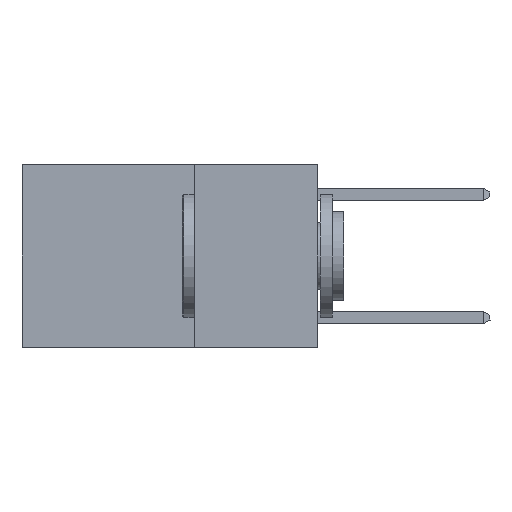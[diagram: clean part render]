
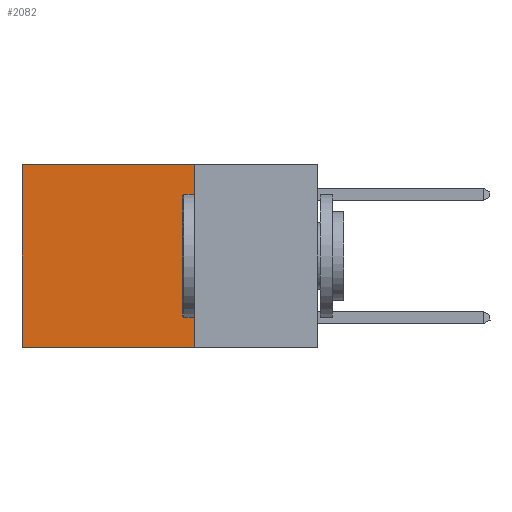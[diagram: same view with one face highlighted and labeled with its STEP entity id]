
A CAD part, left-side view. The second image highlights one B-rep face of the part: STEP entity #2082.
In plain terms, the highlighted planar face has unit normal (-1, 0, 0).
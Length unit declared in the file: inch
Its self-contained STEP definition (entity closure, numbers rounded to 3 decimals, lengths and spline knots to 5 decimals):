
#251 = DIRECTION ( 'NONE',  ( 0., 0., -1. ) ) ;
#356 = CARTESIAN_POINT ( 'NONE',  ( 0.2625, 0.6, 0. ) ) ;
#1364 = ORIENTED_EDGE ( 'NONE', *, *, #13671, .T. ) ;
#1718 = AXIS2_PLACEMENT_3D ( 'NONE', #10897, #9936, #9762 ) ;
#1828 = ORIENTED_EDGE ( 'NONE', *, *, #12898, .F. ) ;
#2082 = ADVANCED_FACE ( 'NONE', ( #7161 ), #16792, .F. ) ;
#2139 = EDGE_CURVE ( 'NONE', #4637, #15109, #13131, .T. ) ;
#2626 = EDGE_CURVE ( 'NONE', #5519, #4915, #13304, .T. ) ;
#2688 = VECTOR ( 'NONE', #3505, 39.37008 ) ;
#2850 = CARTESIAN_POINT ( 'NONE',  ( 0.2625, 0.25, 0. ) ) ;
#3505 = DIRECTION ( 'NONE',  ( 0., 1., 0. ) ) ;
#3754 = DIRECTION ( 'NONE',  ( 0., 1., 0. ) ) ;
#3879 = CARTESIAN_POINT ( 'NONE',  ( 0.2625, 0.25, 0. ) ) ;
#4637 = VERTEX_POINT ( 'NONE', #8286 ) ;
#4915 = VERTEX_POINT ( 'NONE', #356 ) ;
#5519 = VERTEX_POINT ( 'NONE', #2850 ) ;
#5584 = VECTOR ( 'NONE', #251, 39.37008 ) ;
#7161 = FACE_OUTER_BOUND ( 'NONE', #12252, .T. ) ;
#8125 = CARTESIAN_POINT ( 'NONE',  ( 0.2625, 0.6, -0.37 ) ) ;
#8286 = CARTESIAN_POINT ( 'NONE',  ( 0.2625, 0.25, -0.37 ) ) ;
#8288 = VECTOR ( 'NONE', #12950, 39.37008 ) ;
#9135 = LINE ( 'NONE', #14086, #5584 ) ;
#9658 = VECTOR ( 'NONE', #3754, 39.37008 ) ;
#9762 = DIRECTION ( 'NONE',  ( 0., 0., -1. ) ) ;
#9936 = DIRECTION ( 'NONE',  ( 1., 0., 0. ) ) ;
#10897 = CARTESIAN_POINT ( 'NONE',  ( 0.2625, 0.25, 0. ) ) ;
#12252 = EDGE_LOOP ( 'NONE', ( #1364, #12342, #1828, #12774 ) ) ;
#12342 = ORIENTED_EDGE ( 'NONE', *, *, #2139, .F. ) ;
#12717 = CARTESIAN_POINT ( 'NONE',  ( 0.2625, 0.25, -0.37 ) ) ;
#12774 = ORIENTED_EDGE ( 'NONE', *, *, #2626, .T. ) ;
#12898 = EDGE_CURVE ( 'NONE', #5519, #4637, #9135, .T. ) ;
#12950 = DIRECTION ( 'NONE',  ( 0., 0., -1. ) ) ;
#13131 = LINE ( 'NONE', #12717, #2688 ) ;
#13304 = LINE ( 'NONE', #3879, #9658 ) ;
#13671 = EDGE_CURVE ( 'NONE', #4915, #15109, #15822, .T. ) ;
#14086 = CARTESIAN_POINT ( 'NONE',  ( 0.2625, 0.25, 0. ) ) ;
#15109 = VERTEX_POINT ( 'NONE', #8125 ) ;
#15544 = CARTESIAN_POINT ( 'NONE',  ( 0.2625, 0.6, 0. ) ) ;
#15822 = LINE ( 'NONE', #15544, #8288 ) ;
#16792 = PLANE ( 'NONE',  #1718 ) ;
